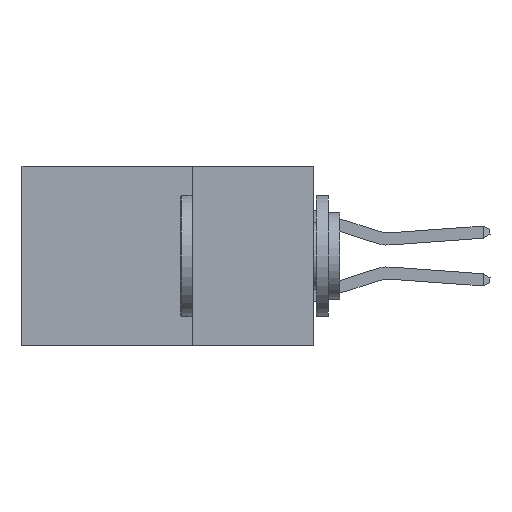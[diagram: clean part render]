
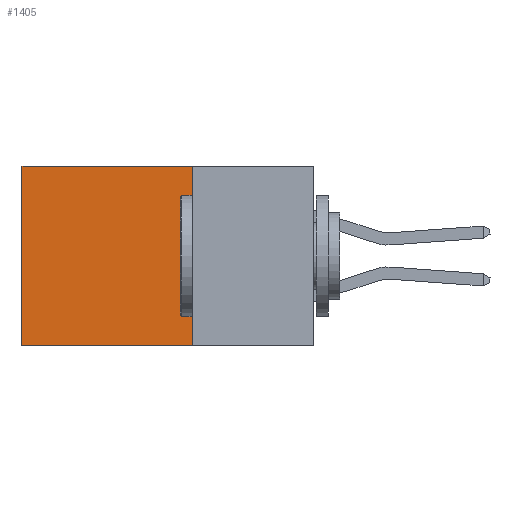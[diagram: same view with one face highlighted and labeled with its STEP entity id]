
A CAD part, left-side view. The second image highlights one B-rep face of the part: STEP entity #1405.
In plain terms, the highlighted planar face has unit normal (-1, 0, 0).
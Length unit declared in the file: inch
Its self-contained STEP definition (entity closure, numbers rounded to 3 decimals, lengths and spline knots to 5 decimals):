
#235 = ORIENTED_EDGE ( 'NONE', *, *, #3217, .T. ) ;
#1280 = ORIENTED_EDGE ( 'NONE', *, *, #14066, .T. ) ;
#1405 = ADVANCED_FACE ( 'NONE', ( #13831 ), #3840, .F. ) ;
#2527 = CARTESIAN_POINT ( 'NONE',  ( 0.2875, 0.25, 0. ) ) ;
#2593 = EDGE_CURVE ( 'NONE', #11113, #14797, #4657, .T. ) ;
#2832 = VERTEX_POINT ( 'NONE', #3095 ) ;
#2853 = LINE ( 'NONE', #14366, #9539 ) ;
#3095 = CARTESIAN_POINT ( 'NONE',  ( 0.2875, 0.6, 0. ) ) ;
#3217 = EDGE_CURVE ( 'NONE', #5403, #2832, #2853, .T. ) ;
#3500 = DIRECTION ( 'NONE',  ( 0., 0., -1. ) ) ;
#3840 = PLANE ( 'NONE',  #16083 ) ;
#4414 = LINE ( 'NONE', #8136, #14153 ) ;
#4654 = CARTESIAN_POINT ( 'NONE',  ( 0.2875, 0.6, -0.37 ) ) ;
#4657 = LINE ( 'NONE', #9484, #11169 ) ;
#5403 = VERTEX_POINT ( 'NONE', #15675 ) ;
#5620 = EDGE_CURVE ( 'NONE', #5403, #11113, #10664, .T. ) ;
#5808 = DIRECTION ( 'NONE',  ( 1., 0., 0. ) ) ;
#7287 = VECTOR ( 'NONE', #10445, 39.37008 ) ;
#7875 = CARTESIAN_POINT ( 'NONE',  ( 0.2875, 0.25, 0. ) ) ;
#8136 = CARTESIAN_POINT ( 'NONE',  ( 0.2875, 0.6, 0. ) ) ;
#9403 = DIRECTION ( 'NONE',  ( 0., 0., -1. ) ) ;
#9457 = DIRECTION ( 'NONE',  ( 0., 1., 0. ) ) ;
#9484 = CARTESIAN_POINT ( 'NONE',  ( 0.2875, 0.25, -0.37 ) ) ;
#9539 = VECTOR ( 'NONE', #14334, 39.37008 ) ;
#10323 = ORIENTED_EDGE ( 'NONE', *, *, #5620, .F. ) ;
#10445 = DIRECTION ( 'NONE',  ( 0., 0., -1. ) ) ;
#10664 = LINE ( 'NONE', #7875, #7287 ) ;
#11113 = VERTEX_POINT ( 'NONE', #11649 ) ;
#11169 = VECTOR ( 'NONE', #9457, 39.37008 ) ;
#11649 = CARTESIAN_POINT ( 'NONE',  ( 0.2875, 0.25, -0.37 ) ) ;
#12978 = ORIENTED_EDGE ( 'NONE', *, *, #2593, .F. ) ;
#13277 = EDGE_LOOP ( 'NONE', ( #1280, #12978, #10323, #235 ) ) ;
#13831 = FACE_OUTER_BOUND ( 'NONE', #13277, .T. ) ;
#14066 = EDGE_CURVE ( 'NONE', #2832, #14797, #4414, .T. ) ;
#14153 = VECTOR ( 'NONE', #9403, 39.37008 ) ;
#14334 = DIRECTION ( 'NONE',  ( 0., 1., 0. ) ) ;
#14366 = CARTESIAN_POINT ( 'NONE',  ( 0.2875, 0.25, 0. ) ) ;
#14797 = VERTEX_POINT ( 'NONE', #4654 ) ;
#15675 = CARTESIAN_POINT ( 'NONE',  ( 0.2875, 0.25, 0. ) ) ;
#16083 = AXIS2_PLACEMENT_3D ( 'NONE', #2527, #5808, #3500 ) ;
